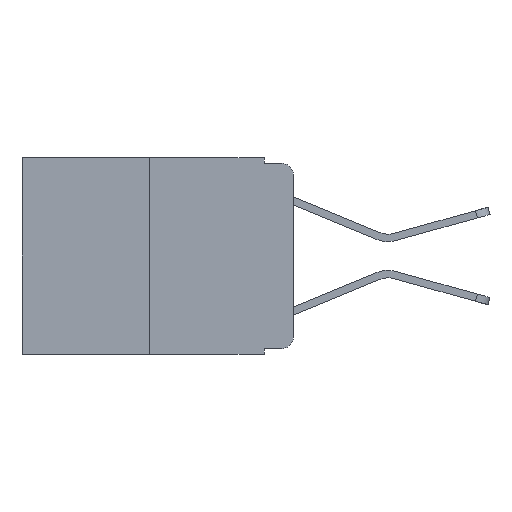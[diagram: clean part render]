
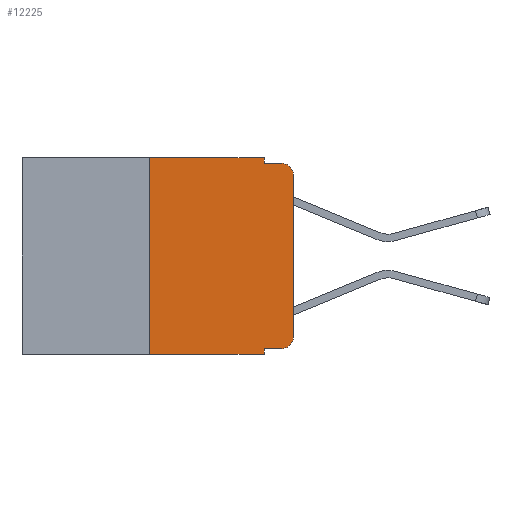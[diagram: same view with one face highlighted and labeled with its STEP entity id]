
A CAD part, left-side view. The second image highlights one B-rep face of the part: STEP entity #12225.
In plain terms, the highlighted planar face has unit normal (-1, 0, 0).
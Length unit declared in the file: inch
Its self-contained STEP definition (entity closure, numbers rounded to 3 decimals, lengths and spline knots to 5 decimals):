
#106 = VERTEX_POINT ( 'NONE', #15885 ) ;
#386 = ORIENTED_EDGE ( 'NONE', *, *, #15917, .F. ) ;
#499 = CARTESIAN_POINT ( 'NONE',  ( 0., 0.051, 0. ) ) ;
#777 = AXIS2_PLACEMENT_3D ( 'NONE', #13587, #6380, #14799 ) ;
#797 = EDGE_CURVE ( 'NONE', #16011, #10213, #3470, .T. ) ;
#948 = DIRECTION ( 'NONE',  ( 0., -1., 0. ) ) ;
#1029 = VERTEX_POINT ( 'NONE', #4711 ) ;
#1727 = EDGE_CURVE ( 'NONE', #1029, #10213, #2287, .T. ) ;
#1782 = DIRECTION ( 'NONE',  ( 0., 0., 1. ) ) ;
#1836 = DIRECTION ( 'NONE',  ( 0., 0., -1. ) ) ;
#2237 = CARTESIAN_POINT ( 'NONE',  ( 0., 0.473, 0. ) ) ;
#2287 = CIRCLE ( 'NONE', #12014, 0.02 ) ;
#2519 = LINE ( 'NONE', #2237, #15117 ) ;
#2572 = EDGE_CURVE ( 'NONE', #4243, #1029, #14032, .T. ) ;
#2870 = CARTESIAN_POINT ( 'NONE',  ( 0., 0., -0.313 ) ) ;
#2878 = VECTOR ( 'NONE', #9684, 39.37008 ) ;
#3080 = VECTOR ( 'NONE', #7890, 39.37008 ) ;
#3470 = LINE ( 'NONE', #11126, #3080 ) ;
#3598 = ORIENTED_EDGE ( 'NONE', *, *, #12729, .T. ) ;
#3797 = ORIENTED_EDGE ( 'NONE', *, *, #15546, .F. ) ;
#3936 = ORIENTED_EDGE ( 'NONE', *, *, #15146, .F. ) ;
#3953 = DIRECTION ( 'NONE',  ( 0., -1., 0. ) ) ;
#4003 = ORIENTED_EDGE ( 'NONE', *, *, #13529, .T. ) ;
#4007 = CARTESIAN_POINT ( 'NONE',  ( 0., 0., 0. ) ) ;
#4243 = VERTEX_POINT ( 'NONE', #2870 ) ;
#4711 = CARTESIAN_POINT ( 'NONE',  ( 0., 0., -0.03 ) ) ;
#4792 = EDGE_CURVE ( 'NONE', #13892, #106, #15841, .T. ) ;
#4866 = PLANE ( 'NONE',  #9812 ) ;
#5335 = VERTEX_POINT ( 'NONE', #14559 ) ;
#5712 = VERTEX_POINT ( 'NONE', #6846 ) ;
#5897 = CARTESIAN_POINT ( 'NONE',  ( 0., 0.25, -0.343 ) ) ;
#5990 = CARTESIAN_POINT ( 'NONE',  ( 0., 0.473, -0.343 ) ) ;
#6078 = VERTEX_POINT ( 'NONE', #13689 ) ;
#6143 = DIRECTION ( 'NONE',  ( 1., 0., 0. ) ) ;
#6309 = LINE ( 'NONE', #12880, #9215 ) ;
#6380 = DIRECTION ( 'NONE',  ( -1., 0., 0. ) ) ;
#6695 = VECTOR ( 'NONE', #3953, 39.37008 ) ;
#6846 = CARTESIAN_POINT ( 'NONE',  ( 0., 0.051, 0. ) ) ;
#7890 = DIRECTION ( 'NONE',  ( 0., -1., 0. ) ) ;
#7943 = ORIENTED_EDGE ( 'NONE', *, *, #2572, .T. ) ;
#8089 = VECTOR ( 'NONE', #1782, 39.37008 ) ;
#8248 = LINE ( 'NONE', #13737, #11011 ) ;
#8603 = CARTESIAN_POINT ( 'NONE',  ( 0., 0.473, 0. ) ) ;
#8884 = CARTESIAN_POINT ( 'NONE',  ( 0., 0.25, 0. ) ) ;
#9215 = VECTOR ( 'NONE', #1836, 39.37008 ) ;
#9684 = DIRECTION ( 'NONE',  ( 0., -1., 0. ) ) ;
#9812 = AXIS2_PLACEMENT_3D ( 'NONE', #8603, #6143, #14554 ) ;
#9920 = LINE ( 'NONE', #12461, #6695 ) ;
#10137 = FACE_OUTER_BOUND ( 'NONE', #10966, .T. ) ;
#10213 = VERTEX_POINT ( 'NONE', #12202 ) ;
#10248 = ORIENTED_EDGE ( 'NONE', *, *, #14320, .F. ) ;
#10400 = CARTESIAN_POINT ( 'NONE',  ( 0., 0.02, -0.03 ) ) ;
#10600 = DIRECTION ( 'NONE',  ( 0., 0., -1. ) ) ;
#10614 = DIRECTION ( 'NONE',  ( -1., 0., 0. ) ) ;
#10621 = LINE ( 'NONE', #499, #13033 ) ;
#10704 = CARTESIAN_POINT ( 'NONE',  ( 0., 0.051, -0.01 ) ) ;
#10966 = EDGE_LOOP ( 'NONE', ( #7943, #15926, #13846, #386, #3797, #3936, #11913, #10248, #4003, #3598 ) ) ;
#11011 = VECTOR ( 'NONE', #12582, 39.37008 ) ;
#11126 = CARTESIAN_POINT ( 'NONE',  ( 0., 0.051, -0.01 ) ) ;
#11913 = ORIENTED_EDGE ( 'NONE', *, *, #4792, .T. ) ;
#12014 = AXIS2_PLACEMENT_3D ( 'NONE', #10400, #10614, #10600 ) ;
#12202 = CARTESIAN_POINT ( 'NONE',  ( 0., 0.02, -0.01 ) ) ;
#12225 = ADVANCED_FACE ( 'NONE', ( #10137 ), #4866, .F. ) ;
#12461 = CARTESIAN_POINT ( 'NONE',  ( 0., 0.051, -0.333 ) ) ;
#12582 = DIRECTION ( 'NONE',  ( 0., 0., 1. ) ) ;
#12729 = EDGE_CURVE ( 'NONE', #6078, #4243, #13311, .T. ) ;
#12736 = VERTEX_POINT ( 'NONE', #8884 ) ;
#12880 = CARTESIAN_POINT ( 'NONE',  ( 0., 0.051, 0. ) ) ;
#13033 = VECTOR ( 'NONE', #15346, 39.37008 ) ;
#13311 = CIRCLE ( 'NONE', #777, 0.02 ) ;
#13529 = EDGE_CURVE ( 'NONE', #5335, #6078, #9920, .T. ) ;
#13587 = CARTESIAN_POINT ( 'NONE',  ( 0., 0.02, -0.313 ) ) ;
#13689 = CARTESIAN_POINT ( 'NONE',  ( 0., 0.02, -0.333 ) ) ;
#13737 = CARTESIAN_POINT ( 'NONE',  ( 0., 0.25, 0. ) ) ;
#13846 = ORIENTED_EDGE ( 'NONE', *, *, #797, .F. ) ;
#13892 = VERTEX_POINT ( 'NONE', #5897 ) ;
#14032 = LINE ( 'NONE', #4007, #8089 ) ;
#14320 = EDGE_CURVE ( 'NONE', #5335, #106, #6309, .T. ) ;
#14554 = DIRECTION ( 'NONE',  ( 0., 0., -1. ) ) ;
#14559 = CARTESIAN_POINT ( 'NONE',  ( 0., 0.051, -0.333 ) ) ;
#14799 = DIRECTION ( 'NONE',  ( 0., 0., -1. ) ) ;
#15117 = VECTOR ( 'NONE', #948, 39.37008 ) ;
#15146 = EDGE_CURVE ( 'NONE', #13892, #12736, #8248, .T. ) ;
#15346 = DIRECTION ( 'NONE',  ( 0., 0., -1. ) ) ;
#15546 = EDGE_CURVE ( 'NONE', #12736, #5712, #2519, .T. ) ;
#15841 = LINE ( 'NONE', #5990, #2878 ) ;
#15885 = CARTESIAN_POINT ( 'NONE',  ( 0., 0.051, -0.343 ) ) ;
#15917 = EDGE_CURVE ( 'NONE', #5712, #16011, #10621, .T. ) ;
#15926 = ORIENTED_EDGE ( 'NONE', *, *, #1727, .T. ) ;
#16011 = VERTEX_POINT ( 'NONE', #10704 ) ;
